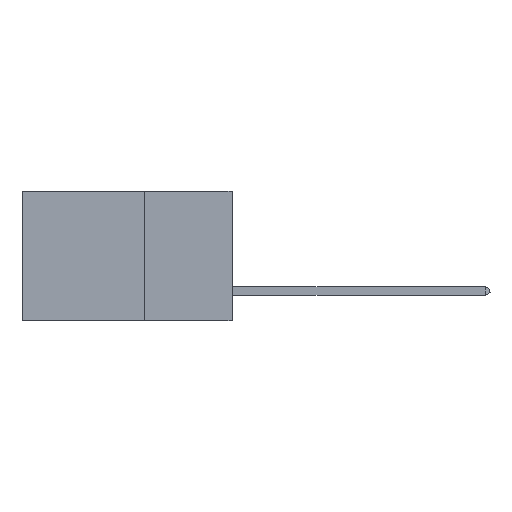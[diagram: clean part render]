
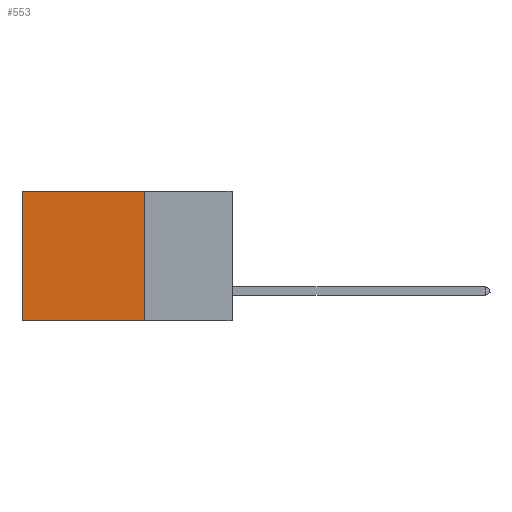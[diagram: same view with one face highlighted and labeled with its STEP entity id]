
A CAD part, left-side view. The second image highlights one B-rep face of the part: STEP entity #553.
In plain terms, the highlighted planar face has unit normal (-1, 0, 0).
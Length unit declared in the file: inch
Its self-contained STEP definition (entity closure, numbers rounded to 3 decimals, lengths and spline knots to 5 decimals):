
#225 = ORIENTED_EDGE ( 'NONE', *, *, #13904, .F. ) ;
#553 = ADVANCED_FACE ( 'NONE', ( #2500 ), #13459, .F. ) ;
#809 = VECTOR ( 'NONE', #4010, 39.37008 ) ;
#1242 = EDGE_CURVE ( 'NONE', #12802, #2227, #3093, .T. ) ;
#1421 = DIRECTION ( 'NONE',  ( 0., 1., 0. ) ) ;
#1551 = ORIENTED_EDGE ( 'NONE', *, *, #6265, .T. ) ;
#2183 = VECTOR ( 'NONE', #3389, 39.37008 ) ;
#2227 = VERTEX_POINT ( 'NONE', #14830 ) ;
#2500 = FACE_OUTER_BOUND ( 'NONE', #3376, .T. ) ;
#3093 = LINE ( 'NONE', #17359, #809 ) ;
#3376 = EDGE_LOOP ( 'NONE', ( #1551, #5558, #225, #5663 ) ) ;
#3389 = DIRECTION ( 'NONE',  ( 0., 0., -1. ) ) ;
#3664 = VECTOR ( 'NONE', #12650, 39.37008 ) ;
#4010 = DIRECTION ( 'NONE',  ( 0., 1., 0. ) ) ;
#4622 = CARTESIAN_POINT ( 'NONE',  ( 0.2875, 0.25, 0. ) ) ;
#5126 = CARTESIAN_POINT ( 'NONE',  ( 0.2875, 0.25, 0. ) ) ;
#5392 = CARTESIAN_POINT ( 'NONE',  ( 0.2875, 0.25, -0.37 ) ) ;
#5425 = LINE ( 'NONE', #5392, #11666 ) ;
#5558 = ORIENTED_EDGE ( 'NONE', *, *, #10638, .F. ) ;
#5663 = ORIENTED_EDGE ( 'NONE', *, *, #1242, .T. ) ;
#6265 = EDGE_CURVE ( 'NONE', #2227, #17301, #11539, .T. ) ;
#7276 = CARTESIAN_POINT ( 'NONE',  ( 0.2875, 0.6, 0. ) ) ;
#9724 = CARTESIAN_POINT ( 'NONE',  ( 0.2875, 0.6, -0.37 ) ) ;
#9912 = VERTEX_POINT ( 'NONE', #12338 ) ;
#10592 = CARTESIAN_POINT ( 'NONE',  ( 0.2875, 0.25, 0. ) ) ;
#10638 = EDGE_CURVE ( 'NONE', #9912, #17301, #5425, .T. ) ;
#11539 = LINE ( 'NONE', #7276, #2183 ) ;
#11570 = AXIS2_PLACEMENT_3D ( 'NONE', #10592, #11927, #13634 ) ;
#11666 = VECTOR ( 'NONE', #1421, 39.37008 ) ;
#11927 = DIRECTION ( 'NONE',  ( 1., 0., 0. ) ) ;
#12338 = CARTESIAN_POINT ( 'NONE',  ( 0.2875, 0.25, -0.37 ) ) ;
#12650 = DIRECTION ( 'NONE',  ( 0., 0., -1. ) ) ;
#12802 = VERTEX_POINT ( 'NONE', #5126 ) ;
#13459 = PLANE ( 'NONE',  #11570 ) ;
#13634 = DIRECTION ( 'NONE',  ( 0., 0., -1. ) ) ;
#13904 = EDGE_CURVE ( 'NONE', #12802, #9912, #16648, .T. ) ;
#14830 = CARTESIAN_POINT ( 'NONE',  ( 0.2875, 0.6, 0. ) ) ;
#16648 = LINE ( 'NONE', #4622, #3664 ) ;
#17301 = VERTEX_POINT ( 'NONE', #9724 ) ;
#17359 = CARTESIAN_POINT ( 'NONE',  ( 0.2875, 0.25, 0. ) ) ;
